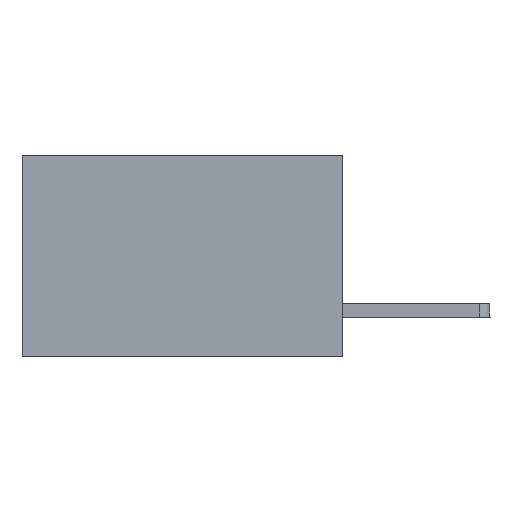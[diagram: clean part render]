
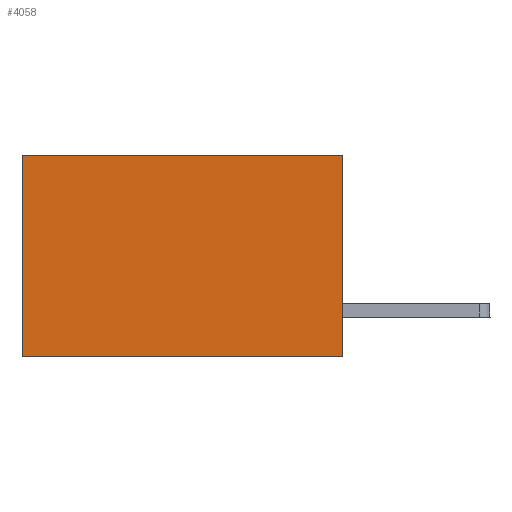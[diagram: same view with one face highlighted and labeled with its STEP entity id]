
A CAD part, left-side view. The second image highlights one B-rep face of the part: STEP entity #4058.
In plain terms, the highlighted planar face has unit normal (-1, 0, 0).
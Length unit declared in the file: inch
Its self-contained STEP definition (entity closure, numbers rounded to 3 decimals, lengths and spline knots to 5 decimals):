
#223 = DIRECTION ( 'NONE',  ( 0., 1., 0. ) ) ;
#563 = EDGE_CURVE ( 'NONE', #3033, #9161, #2273, .T. ) ;
#681 = CARTESIAN_POINT ( 'NONE',  ( 0.277, 0., -0.37 ) ) ;
#1096 = EDGE_CURVE ( 'NONE', #4338, #9161, #13021, .T. ) ;
#1362 = EDGE_CURVE ( 'NONE', #13208, #3033, #8459, .T. ) ;
#1783 = VECTOR ( 'NONE', #3776, 39.37008 ) ;
#2071 = ORIENTED_EDGE ( 'NONE', *, *, #9405, .T. ) ;
#2162 = DIRECTION ( 'NONE',  ( 0., 0., -1. ) ) ;
#2273 = LINE ( 'NONE', #3448, #4263 ) ;
#2335 = ORIENTED_EDGE ( 'NONE', *, *, #563, .F. ) ;
#2827 = FACE_OUTER_BOUND ( 'NONE', #8268, .T. ) ;
#3033 = VERTEX_POINT ( 'NONE', #681 ) ;
#3200 = CARTESIAN_POINT ( 'NONE',  ( 0.277, 0., -0.37 ) ) ;
#3385 = VECTOR ( 'NONE', #223, 39.37008 ) ;
#3448 = CARTESIAN_POINT ( 'NONE',  ( 0.277, 0., -0.37 ) ) ;
#3488 = CARTESIAN_POINT ( 'NONE',  ( 0.277, 0.59, 0. ) ) ;
#3776 = DIRECTION ( 'NONE',  ( 0., 0., -1. ) ) ;
#4058 = ADVANCED_FACE ( 'NONE', ( #2827 ), #5873, .F. ) ;
#4263 = VECTOR ( 'NONE', #7657, 39.37008 ) ;
#4338 = VERTEX_POINT ( 'NONE', #3488 ) ;
#4567 = LINE ( 'NONE', #8777, #3385 ) ;
#5345 = ORIENTED_EDGE ( 'NONE', *, *, #1362, .F. ) ;
#5873 = PLANE ( 'NONE',  #11547 ) ;
#6534 = ORIENTED_EDGE ( 'NONE', *, *, #1096, .T. ) ;
#6610 = CARTESIAN_POINT ( 'NONE',  ( 0.277, 0.59, -0.37 ) ) ;
#6751 = CARTESIAN_POINT ( 'NONE',  ( 0.277, 0.59, -0.37 ) ) ;
#6913 = CARTESIAN_POINT ( 'NONE',  ( 0.277, 0., -0.37 ) ) ;
#7657 = DIRECTION ( 'NONE',  ( 0., 1., 0. ) ) ;
#8268 = EDGE_LOOP ( 'NONE', ( #6534, #2335, #5345, #2071 ) ) ;
#8459 = LINE ( 'NONE', #3200, #12739 ) ;
#8777 = CARTESIAN_POINT ( 'NONE',  ( 0.277, 0., 0. ) ) ;
#9161 = VERTEX_POINT ( 'NONE', #6610 ) ;
#9405 = EDGE_CURVE ( 'NONE', #13208, #4338, #4567, .T. ) ;
#10741 = CARTESIAN_POINT ( 'NONE',  ( 0.277, 0., 0. ) ) ;
#11547 = AXIS2_PLACEMENT_3D ( 'NONE', #6913, #13261, #13330 ) ;
#12739 = VECTOR ( 'NONE', #2162, 39.37008 ) ;
#13021 = LINE ( 'NONE', #6751, #1783 ) ;
#13208 = VERTEX_POINT ( 'NONE', #10741 ) ;
#13261 = DIRECTION ( 'NONE',  ( 1., 0., 0. ) ) ;
#13330 = DIRECTION ( 'NONE',  ( 0., 0., -1. ) ) ;
